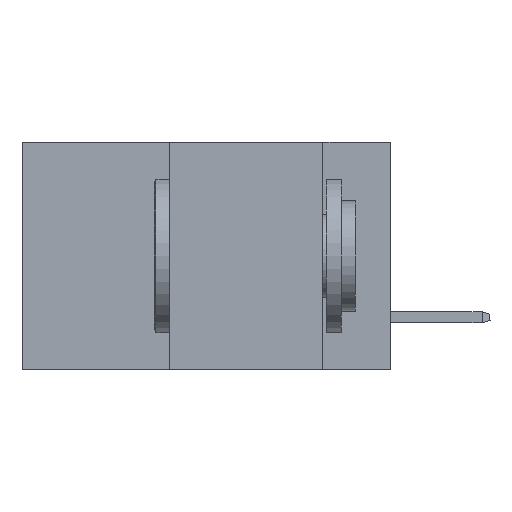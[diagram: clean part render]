
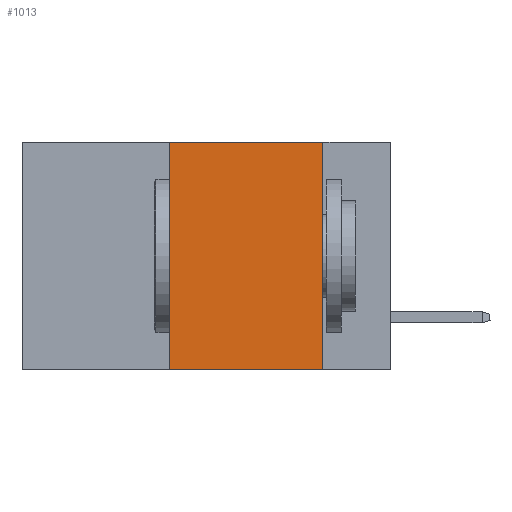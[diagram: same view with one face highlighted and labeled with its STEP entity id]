
A CAD part, left-side view. The second image highlights one B-rep face of the part: STEP entity #1013.
In plain terms, the highlighted planar face has unit normal (-1, 0, 0).
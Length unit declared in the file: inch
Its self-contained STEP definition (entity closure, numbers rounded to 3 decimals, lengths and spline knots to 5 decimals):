
#2 = ORIENTED_EDGE ( 'NONE', *, *, #16130, .T. ) ;
#500 = VECTOR ( 'NONE', #3255, 39.37008 ) ;
#705 = VERTEX_POINT ( 'NONE', #23088 ) ;
#844 = VECTOR ( 'NONE', #8065, 39.37008 ) ;
#1013 = ADVANCED_FACE ( 'NONE', ( #2979 ), #12552, .F. ) ;
#2834 = CARTESIAN_POINT ( 'NONE',  ( 0., 0.11, 0. ) ) ;
#2979 = FACE_OUTER_BOUND ( 'NONE', #18034, .T. ) ;
#2990 = CARTESIAN_POINT ( 'NONE',  ( 0., 0.6, 0. ) ) ;
#3088 = LINE ( 'NONE', #2834, #23980 ) ;
#3255 = DIRECTION ( 'NONE',  ( 0., -1., 0. ) ) ;
#4182 = AXIS2_PLACEMENT_3D ( 'NONE', #2990, #14744, #16659 ) ;
#4918 = DIRECTION ( 'NONE',  ( 0., 0., -1. ) ) ;
#5623 = DIRECTION ( 'NONE',  ( 0., 0., 1. ) ) ;
#6070 = CARTESIAN_POINT ( 'NONE',  ( 0., 0.6, -0.37 ) ) ;
#7574 = EDGE_CURVE ( 'NONE', #705, #22927, #15616, .T. ) ;
#7620 = VERTEX_POINT ( 'NONE', #9640 ) ;
#8065 = DIRECTION ( 'NONE',  ( 0., -1., 0. ) ) ;
#9640 = CARTESIAN_POINT ( 'NONE',  ( 0., 0.11, -0.37 ) ) ;
#11938 = VERTEX_POINT ( 'NONE', #12646 ) ;
#11947 = CARTESIAN_POINT ( 'NONE',  ( 0., 0.11, 0. ) ) ;
#12552 = PLANE ( 'NONE',  #4182 ) ;
#12646 = CARTESIAN_POINT ( 'NONE',  ( 0., 0.36, -0.37 ) ) ;
#14030 = EDGE_CURVE ( 'NONE', #22927, #7620, #3088, .T. ) ;
#14744 = DIRECTION ( 'NONE',  ( 1., 0., 0. ) ) ;
#15616 = LINE ( 'NONE', #22319, #500 ) ;
#16072 = EDGE_CURVE ( 'NONE', #11938, #705, #17474, .T. ) ;
#16130 = EDGE_CURVE ( 'NONE', #11938, #7620, #23000, .T. ) ;
#16659 = DIRECTION ( 'NONE',  ( 0., 0., -1. ) ) ;
#17202 = CARTESIAN_POINT ( 'NONE',  ( 0., 0.36, 0. ) ) ;
#17474 = LINE ( 'NONE', #17202, #24775 ) ;
#18034 = EDGE_LOOP ( 'NONE', ( #22545, #18435, #18440, #2 ) ) ;
#18435 = ORIENTED_EDGE ( 'NONE', *, *, #7574, .F. ) ;
#18440 = ORIENTED_EDGE ( 'NONE', *, *, #16072, .F. ) ;
#22319 = CARTESIAN_POINT ( 'NONE',  ( 0., 0.6, 0. ) ) ;
#22545 = ORIENTED_EDGE ( 'NONE', *, *, #14030, .F. ) ;
#22927 = VERTEX_POINT ( 'NONE', #11947 ) ;
#23000 = LINE ( 'NONE', #6070, #844 ) ;
#23088 = CARTESIAN_POINT ( 'NONE',  ( 0., 0.36, 0. ) ) ;
#23980 = VECTOR ( 'NONE', #4918, 39.37008 ) ;
#24775 = VECTOR ( 'NONE', #5623, 39.37008 ) ;
